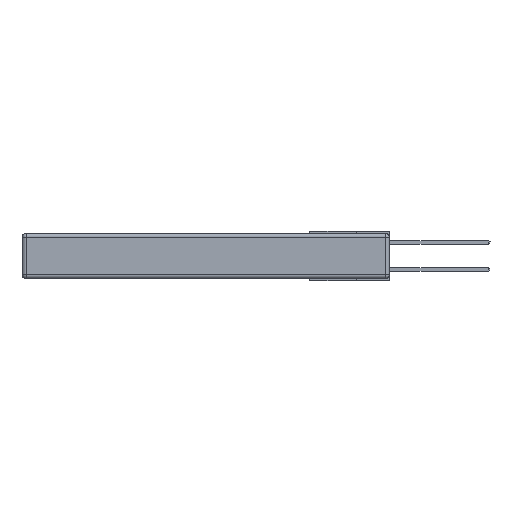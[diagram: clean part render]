
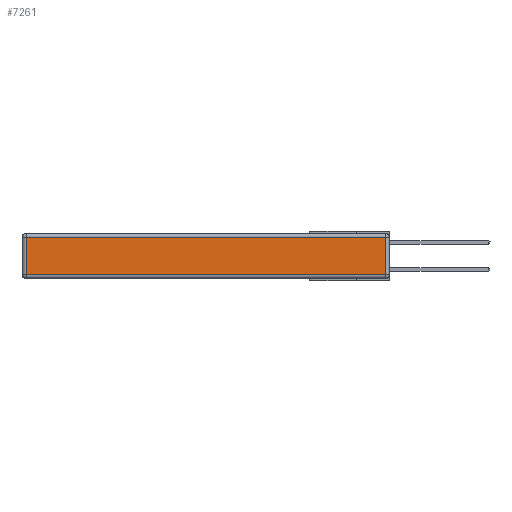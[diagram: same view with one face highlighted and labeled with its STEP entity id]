
A CAD part, left-side view. The second image highlights one B-rep face of the part: STEP entity #7261.
In plain terms, the highlighted planar face has unit normal (-1, 0, 0).
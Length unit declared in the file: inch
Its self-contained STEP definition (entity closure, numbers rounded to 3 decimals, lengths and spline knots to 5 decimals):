
#807 = EDGE_CURVE ( 'NONE', #18164, #1552, #9176, .T. ) ;
#1552 = VERTEX_POINT ( 'NONE', #14093 ) ;
#1593 = DIRECTION ( 'NONE',  ( 0., 0., -1. ) ) ;
#2760 = EDGE_CURVE ( 'NONE', #1552, #23113, #9308, .T. ) ;
#2922 = DIRECTION ( 'NONE',  ( 0., 0., 1. ) ) ;
#3972 = EDGE_LOOP ( 'NONE', ( #7589, #6149, #13755, #4840 ) ) ;
#4067 = DIRECTION ( 'NONE',  ( -1., 0., 0. ) ) ;
#4724 = CARTESIAN_POINT ( 'NONE',  ( 0., 2.75, -0.03 ) ) ;
#4840 = ORIENTED_EDGE ( 'NONE', *, *, #2760, .T. ) ;
#5088 = LINE ( 'NONE', #12104, #19175 ) ;
#5553 = EDGE_CURVE ( 'NONE', #23113, #16124, #12674, .T. ) ;
#6149 = ORIENTED_EDGE ( 'NONE', *, *, #21773, .T. ) ;
#7051 = DIRECTION ( 'NONE',  ( 0., -1., 0. ) ) ;
#7261 = ADVANCED_FACE ( 'NONE', ( #11445 ), #14874, .T. ) ;
#7589 = ORIENTED_EDGE ( 'NONE', *, *, #5553, .T. ) ;
#7684 = CARTESIAN_POINT ( 'NONE',  ( 0., 0., -0.343 ) ) ;
#7750 = VECTOR ( 'NONE', #7051, 39.37008 ) ;
#7764 = DIRECTION ( 'NONE',  ( 0., 0., 1. ) ) ;
#9013 = CARTESIAN_POINT ( 'NONE',  ( 0., 2.72, -0.343 ) ) ;
#9176 = LINE ( 'NONE', #4724, #22408 ) ;
#9308 = LINE ( 'NONE', #9013, #9603 ) ;
#9603 = VECTOR ( 'NONE', #1593, 39.37008 ) ;
#11445 = FACE_OUTER_BOUND ( 'NONE', #3972, .T. ) ;
#11448 = CARTESIAN_POINT ( 'NONE',  ( 0., 0.03, -0.03 ) ) ;
#11856 = CARTESIAN_POINT ( 'NONE',  ( 0., 2.72, -0.313 ) ) ;
#12104 = CARTESIAN_POINT ( 'NONE',  ( 0., 0.03, -0.343 ) ) ;
#12674 = LINE ( 'NONE', #13975, #7750 ) ;
#13755 = ORIENTED_EDGE ( 'NONE', *, *, #807, .T. ) ;
#13975 = CARTESIAN_POINT ( 'NONE',  ( 0., 0., -0.313 ) ) ;
#14093 = CARTESIAN_POINT ( 'NONE',  ( 0., 2.72, -0.03 ) ) ;
#14539 = AXIS2_PLACEMENT_3D ( 'NONE', #7684, #4067, #7764 ) ;
#14874 = PLANE ( 'NONE',  #14539 ) ;
#16123 = CARTESIAN_POINT ( 'NONE',  ( 0., 0.03, -0.313 ) ) ;
#16124 = VERTEX_POINT ( 'NONE', #16123 ) ;
#17780 = DIRECTION ( 'NONE',  ( 0., 1., 0. ) ) ;
#18164 = VERTEX_POINT ( 'NONE', #11448 ) ;
#19175 = VECTOR ( 'NONE', #2922, 39.37008 ) ;
#21773 = EDGE_CURVE ( 'NONE', #16124, #18164, #5088, .T. ) ;
#22408 = VECTOR ( 'NONE', #17780, 39.37008 ) ;
#23113 = VERTEX_POINT ( 'NONE', #11856 ) ;
